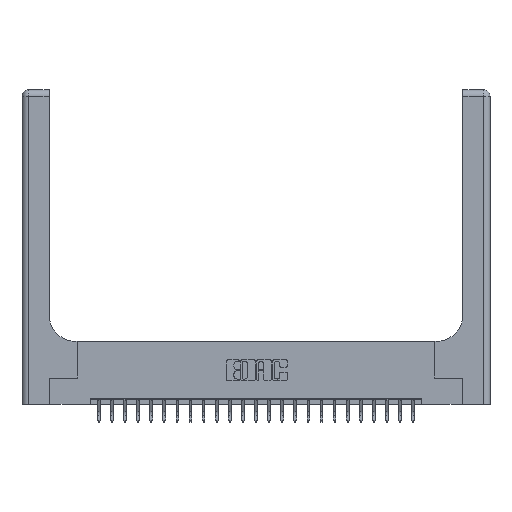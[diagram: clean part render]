
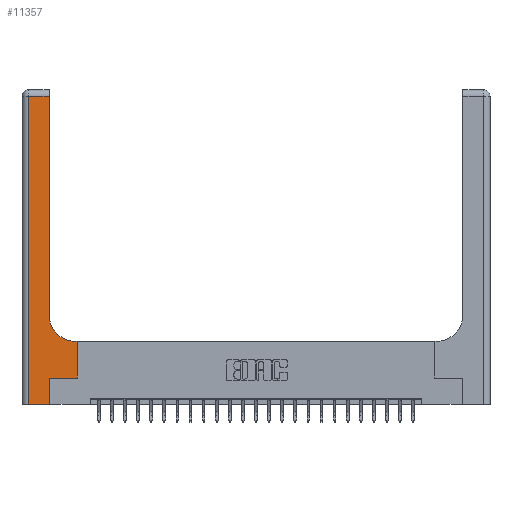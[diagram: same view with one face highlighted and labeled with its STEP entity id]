
A CAD part, top view. The second image highlights one B-rep face of the part: STEP entity #11357.
In plain terms, the highlighted planar face has unit normal (0, 0, 1).
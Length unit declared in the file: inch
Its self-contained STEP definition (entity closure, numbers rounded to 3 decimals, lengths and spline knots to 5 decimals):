
#100 = CARTESIAN_POINT ( 'NONE',  ( 0.26, 0.6, 0.37 ) ) ;
#334 = VERTEX_POINT ( 'NONE', #2985 ) ;
#1264 = LINE ( 'NONE', #14354, #14829 ) ;
#1450 = DIRECTION ( 'NONE',  ( 0., 1., 0. ) ) ;
#2002 = ORIENTED_EDGE ( 'NONE', *, *, #7547, .T. ) ;
#2190 = AXIS2_PLACEMENT_3D ( 'NONE', #11711, #11010, #16828 ) ;
#2394 = LINE ( 'NONE', #11672, #17515 ) ;
#2613 = CARTESIAN_POINT ( 'NONE',  ( 0.265, 0.25, 0.37 ) ) ;
#2844 = VERTEX_POINT ( 'NONE', #10174 ) ;
#2851 = ORIENTED_EDGE ( 'NONE', *, *, #11461, .T. ) ;
#2985 = CARTESIAN_POINT ( 'NONE',  ( 0.26, 0.85, 0.37 ) ) ;
#3050 = CARTESIAN_POINT ( 'NONE',  ( 0.06, 2.94, 0.37 ) ) ;
#3292 = CARTESIAN_POINT ( 'NONE',  ( 0.528, 0.25, 0.37 ) ) ;
#3685 = PLANE ( 'NONE',  #19155 ) ;
#3713 = ORIENTED_EDGE ( 'NONE', *, *, #5188, .T. ) ;
#4144 = EDGE_CURVE ( 'NONE', #6908, #2844, #7990, .T. ) ;
#4265 = CARTESIAN_POINT ( 'NONE',  ( 0., 2.94, 0.37 ) ) ;
#5188 = EDGE_CURVE ( 'NONE', #2844, #10991, #12002, .T. ) ;
#5379 = EDGE_CURVE ( 'NONE', #13374, #334, #9728, .T. ) ;
#5637 = CARTESIAN_POINT ( 'NONE',  ( 0.51, 0.6, 0.37 ) ) ;
#5698 = LINE ( 'NONE', #100, #12421 ) ;
#5934 = ORIENTED_EDGE ( 'NONE', *, *, #8820, .T. ) ;
#6141 = DIRECTION ( 'NONE',  ( -1., 0., 0. ) ) ;
#6448 = CARTESIAN_POINT ( 'NONE',  ( 0.06, 0., 0.37 ) ) ;
#6586 = VECTOR ( 'NONE', #1450, 39.37008 ) ;
#6908 = VERTEX_POINT ( 'NONE', #7415 ) ;
#7336 = VECTOR ( 'NONE', #10178, 39.37008 ) ;
#7415 = CARTESIAN_POINT ( 'NONE',  ( 0.265, 0., 0.37 ) ) ;
#7441 = CARTESIAN_POINT ( 'NONE',  ( 0.528, 0.25, 0.37 ) ) ;
#7547 = EDGE_CURVE ( 'NONE', #334, #23301, #1264, .T. ) ;
#7990 = LINE ( 'NONE', #19613, #16763 ) ;
#8670 = VECTOR ( 'NONE', #6141, 39.37008 ) ;
#8750 = EDGE_CURVE ( 'NONE', #21946, #17580, #24211, .T. ) ;
#8812 = DIRECTION ( 'NONE',  ( 0., 1., 0. ) ) ;
#8820 = EDGE_CURVE ( 'NONE', #23301, #21946, #15273, .T. ) ;
#9022 = FACE_OUTER_BOUND ( 'NONE', #22602, .T. ) ;
#9728 = CIRCLE ( 'NONE', #2190, 0.25 ) ;
#9996 = DIRECTION ( 'NONE',  ( -1., 0., 0. ) ) ;
#10174 = CARTESIAN_POINT ( 'NONE',  ( 0.265, 0.25, 0.37 ) ) ;
#10178 = DIRECTION ( 'NONE',  ( 1., 0., 0. ) ) ;
#10991 = VERTEX_POINT ( 'NONE', #7441 ) ;
#11010 = DIRECTION ( 'NONE',  ( 0., 0., -1. ) ) ;
#11318 = DIRECTION ( 'NONE',  ( 0., -1., 0. ) ) ;
#11357 = ADVANCED_FACE ( 'NONE', ( #9022 ), #3685, .F. ) ;
#11461 = EDGE_CURVE ( 'NONE', #15452, #13374, #5698, .T. ) ;
#11672 = CARTESIAN_POINT ( 'NONE',  ( 0., 0., 0.37 ) ) ;
#11711 = CARTESIAN_POINT ( 'NONE',  ( 0.51, 0.85, 0.37 ) ) ;
#12002 = LINE ( 'NONE', #2613, #7336 ) ;
#12421 = VECTOR ( 'NONE', #9996, 39.37008 ) ;
#13162 = DIRECTION ( 'NONE',  ( 1., 0., 0. ) ) ;
#13374 = VERTEX_POINT ( 'NONE', #5637 ) ;
#14354 = CARTESIAN_POINT ( 'NONE',  ( 0.26, 3., 0.37 ) ) ;
#14829 = VECTOR ( 'NONE', #8812, 39.37008 ) ;
#15273 = LINE ( 'NONE', #4265, #8670 ) ;
#15452 = VERTEX_POINT ( 'NONE', #23027 ) ;
#16547 = DIRECTION ( 'NONE',  ( -1., 0., 0. ) ) ;
#16763 = VECTOR ( 'NONE', #22979, 39.37008 ) ;
#16800 = CARTESIAN_POINT ( 'NONE',  ( 0., 3., 0.37 ) ) ;
#16828 = DIRECTION ( 'NONE',  ( 1., 0., 0. ) ) ;
#16921 = DIRECTION ( 'NONE',  ( 0., 0., -1. ) ) ;
#17515 = VECTOR ( 'NONE', #13162, 39.37008 ) ;
#17580 = VERTEX_POINT ( 'NONE', #6448 ) ;
#18389 = LINE ( 'NONE', #3292, #6586 ) ;
#18810 = ORIENTED_EDGE ( 'NONE', *, *, #5379, .T. ) ;
#18953 = VECTOR ( 'NONE', #11318, 39.37008 ) ;
#19155 = AXIS2_PLACEMENT_3D ( 'NONE', #16800, #16921, #16547 ) ;
#19613 = CARTESIAN_POINT ( 'NONE',  ( 0.265, 0., 0.37 ) ) ;
#20029 = ORIENTED_EDGE ( 'NONE', *, *, #4144, .T. ) ;
#20110 = EDGE_CURVE ( 'NONE', #17580, #6908, #2394, .T. ) ;
#20497 = CARTESIAN_POINT ( 'NONE',  ( 0.06, 3., 0.37 ) ) ;
#20704 = ORIENTED_EDGE ( 'NONE', *, *, #20110, .T. ) ;
#21946 = VERTEX_POINT ( 'NONE', #3050 ) ;
#22602 = EDGE_LOOP ( 'NONE', ( #2002, #5934, #22871, #20704, #20029, #3713, #22606, #2851, #18810 ) ) ;
#22606 = ORIENTED_EDGE ( 'NONE', *, *, #23663, .T. ) ;
#22871 = ORIENTED_EDGE ( 'NONE', *, *, #8750, .T. ) ;
#22979 = DIRECTION ( 'NONE',  ( 0., 1., 0. ) ) ;
#23027 = CARTESIAN_POINT ( 'NONE',  ( 0.528, 0.6, 0.37 ) ) ;
#23301 = VERTEX_POINT ( 'NONE', #23366 ) ;
#23366 = CARTESIAN_POINT ( 'NONE',  ( 0.26, 2.94, 0.37 ) ) ;
#23663 = EDGE_CURVE ( 'NONE', #10991, #15452, #18389, .T. ) ;
#24211 = LINE ( 'NONE', #20497, #18953 ) ;
